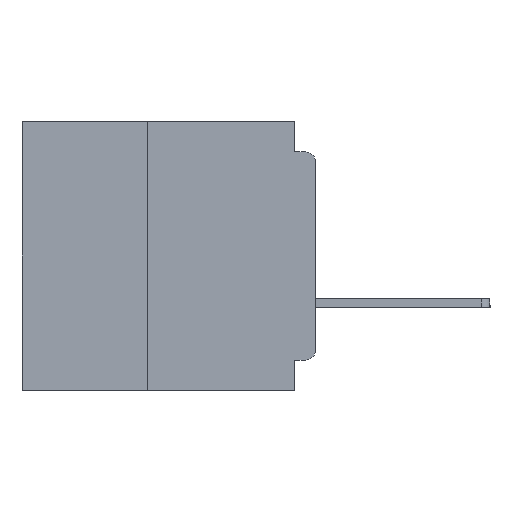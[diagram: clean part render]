
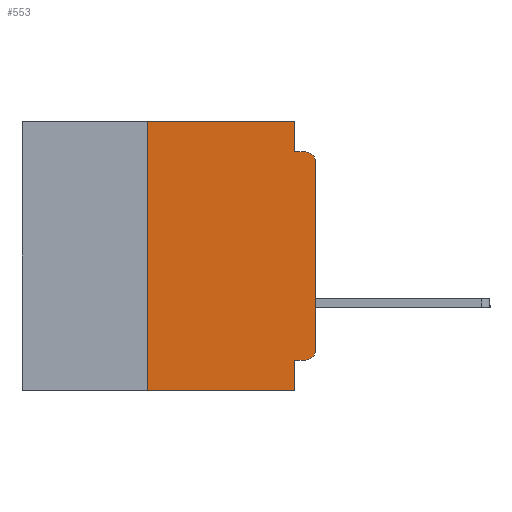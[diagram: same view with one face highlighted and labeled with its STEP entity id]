
A CAD part, left-side view. The second image highlights one B-rep face of the part: STEP entity #553.
In plain terms, the highlighted planar face has unit normal (-1, 0, 0).
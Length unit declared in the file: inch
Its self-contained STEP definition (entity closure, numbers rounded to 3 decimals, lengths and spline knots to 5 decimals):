
#211 = LINE ( 'NONE', #34691, #37572 ) ;
#217 = EDGE_CURVE ( 'NONE', #37705, #14014, #10165, .T. ) ;
#553 = ADVANCED_FACE ( 'NONE', ( #25404 ), #17143, .F. ) ;
#1602 = DIRECTION ( 'NONE',  ( 0., 0., -1. ) ) ;
#2758 = AXIS2_PLACEMENT_3D ( 'NONE', #35565, #41936, #1602 ) ;
#2790 = VERTEX_POINT ( 'NONE', #4789 ) ;
#3664 = CARTESIAN_POINT ( 'NONE',  ( 0., 0.031, -0.355 ) ) ;
#4577 = VECTOR ( 'NONE', #31109, 39.37008 ) ;
#4789 = CARTESIAN_POINT ( 'NONE',  ( 0., 0.015, -0.355 ) ) ;
#5181 = DIRECTION ( 'NONE',  ( 0., 0., -1. ) ) ;
#5462 = VERTEX_POINT ( 'NONE', #20794 ) ;
#5554 = VERTEX_POINT ( 'NONE', #38667 ) ;
#5635 = DIRECTION ( 'NONE',  ( -1., 0., 0. ) ) ;
#5805 = AXIS2_PLACEMENT_3D ( 'NONE', #36623, #15779, #40121 ) ;
#7136 = LINE ( 'NONE', #25974, #15381 ) ;
#7722 = LINE ( 'NONE', #7959, #26225 ) ;
#7959 = CARTESIAN_POINT ( 'NONE',  ( 0., 0.437, -0.4 ) ) ;
#8153 = VERTEX_POINT ( 'NONE', #33661 ) ;
#8829 = CARTESIAN_POINT ( 'NONE',  ( 0., 0.031, -0.4 ) ) ;
#10165 = LINE ( 'NONE', #34430, #44974 ) ;
#10315 = DIRECTION ( 'NONE',  ( 0., 0., 1. ) ) ;
#10323 = DIRECTION ( 'NONE',  ( 0., -1., 0. ) ) ;
#11527 = VERTEX_POINT ( 'NONE', #18605 ) ;
#12233 = ORIENTED_EDGE ( 'NONE', *, *, #217, .F. ) ;
#12251 = EDGE_CURVE ( 'NONE', #21963, #34680, #7136, .T. ) ;
#13641 = CARTESIAN_POINT ( 'NONE',  ( 0., 0., 0. ) ) ;
#14014 = VERTEX_POINT ( 'NONE', #32424 ) ;
#15381 = VECTOR ( 'NONE', #5181, 39.37008 ) ;
#15433 = EDGE_CURVE ( 'NONE', #29196, #5554, #34447, .T. ) ;
#15607 = ORIENTED_EDGE ( 'NONE', *, *, #24206, .F. ) ;
#15779 = DIRECTION ( 'NONE',  ( -1., 0., 0. ) ) ;
#15967 = CARTESIAN_POINT ( 'NONE',  ( 0., 0.031, 0. ) ) ;
#17143 = PLANE ( 'NONE',  #2758 ) ;
#18605 = CARTESIAN_POINT ( 'NONE',  ( 0., 0., -0.06 ) ) ;
#20349 = VECTOR ( 'NONE', #34526, 39.37008 ) ;
#20794 = CARTESIAN_POINT ( 'NONE',  ( 0., 0.015, -0.045 ) ) ;
#20952 = ORIENTED_EDGE ( 'NONE', *, *, #31764, .T. ) ;
#21963 = VERTEX_POINT ( 'NONE', #15967 ) ;
#22730 = EDGE_CURVE ( 'NONE', #2790, #8153, #42563, .T. ) ;
#22908 = DIRECTION ( 'NONE',  ( 0., 0., -1. ) ) ;
#24206 = EDGE_CURVE ( 'NONE', #14014, #21963, #211, .T. ) ;
#24808 = EDGE_CURVE ( 'NONE', #8153, #11527, #25392, .T. ) ;
#25170 = ORIENTED_EDGE ( 'NONE', *, *, #30384, .F. ) ;
#25392 = LINE ( 'NONE', #13641, #4577 ) ;
#25404 = FACE_OUTER_BOUND ( 'NONE', #36204, .T. ) ;
#25576 = ORIENTED_EDGE ( 'NONE', *, *, #15433, .F. ) ;
#25640 = ORIENTED_EDGE ( 'NONE', *, *, #24808, .T. ) ;
#25974 = CARTESIAN_POINT ( 'NONE',  ( 0., 0.031, 0. ) ) ;
#26225 = VECTOR ( 'NONE', #32360, 39.37008 ) ;
#26550 = CARTESIAN_POINT ( 'NONE',  ( 0., 0.015, -0.06 ) ) ;
#26652 = DIRECTION ( 'NONE',  ( 0., 1., 0. ) ) ;
#27622 = CARTESIAN_POINT ( 'NONE',  ( 0., 0.031, -0.045 ) ) ;
#28907 = EDGE_CURVE ( 'NONE', #2790, #29196, #33285, .T. ) ;
#29196 = VERTEX_POINT ( 'NONE', #3664 ) ;
#29486 = CIRCLE ( 'NONE', #35224, 0.015 ) ;
#30090 = DIRECTION ( 'NONE',  ( 0., 0., -1. ) ) ;
#30384 = EDGE_CURVE ( 'NONE', #34680, #5462, #41120, .T. ) ;
#31109 = DIRECTION ( 'NONE',  ( 0., 0., 1. ) ) ;
#31461 = CARTESIAN_POINT ( 'NONE',  ( 0., 0.25, -0.4 ) ) ;
#31764 = EDGE_CURVE ( 'NONE', #37705, #5554, #7722, .T. ) ;
#32193 = VECTOR ( 'NONE', #26652, 39.37008 ) ;
#32360 = DIRECTION ( 'NONE',  ( 0., -1., 0. ) ) ;
#32424 = CARTESIAN_POINT ( 'NONE',  ( 0., 0.25, 0. ) ) ;
#33285 = LINE ( 'NONE', #33582, #32193 ) ;
#33582 = CARTESIAN_POINT ( 'NONE',  ( 0., 0., -0.355 ) ) ;
#33661 = CARTESIAN_POINT ( 'NONE',  ( 0., 0., -0.34 ) ) ;
#34430 = CARTESIAN_POINT ( 'NONE',  ( 0., 0.25, -0.4 ) ) ;
#34447 = LINE ( 'NONE', #8829, #42616 ) ;
#34526 = DIRECTION ( 'NONE',  ( 0., -1., 0. ) ) ;
#34680 = VERTEX_POINT ( 'NONE', #27622 ) ;
#34691 = CARTESIAN_POINT ( 'NONE',  ( 0., 0.437, 0. ) ) ;
#35224 = AXIS2_PLACEMENT_3D ( 'NONE', #26550, #5635, #30090 ) ;
#35565 = CARTESIAN_POINT ( 'NONE',  ( 0., 0.437, 0. ) ) ;
#36204 = EDGE_LOOP ( 'NONE', ( #25640, #41054, #25170, #41782, #15607, #12233, #20952, #25576, #43561, #38762 ) ) ;
#36623 = CARTESIAN_POINT ( 'NONE',  ( 0., 0.015, -0.34 ) ) ;
#37572 = VECTOR ( 'NONE', #10323, 39.37008 ) ;
#37705 = VERTEX_POINT ( 'NONE', #31461 ) ;
#37862 = CARTESIAN_POINT ( 'NONE',  ( 0., 0., -0.045 ) ) ;
#38667 = CARTESIAN_POINT ( 'NONE',  ( 0., 0.031, -0.4 ) ) ;
#38762 = ORIENTED_EDGE ( 'NONE', *, *, #22730, .T. ) ;
#40121 = DIRECTION ( 'NONE',  ( 0., 0., -1. ) ) ;
#41054 = ORIENTED_EDGE ( 'NONE', *, *, #41490, .T. ) ;
#41120 = LINE ( 'NONE', #37862, #20349 ) ;
#41490 = EDGE_CURVE ( 'NONE', #11527, #5462, #29486, .T. ) ;
#41782 = ORIENTED_EDGE ( 'NONE', *, *, #12251, .F. ) ;
#41936 = DIRECTION ( 'NONE',  ( 1., 0., 0. ) ) ;
#42563 = CIRCLE ( 'NONE', #5805, 0.015 ) ;
#42616 = VECTOR ( 'NONE', #22908, 39.37008 ) ;
#43561 = ORIENTED_EDGE ( 'NONE', *, *, #28907, .F. ) ;
#44974 = VECTOR ( 'NONE', #10315, 39.37008 ) ;
